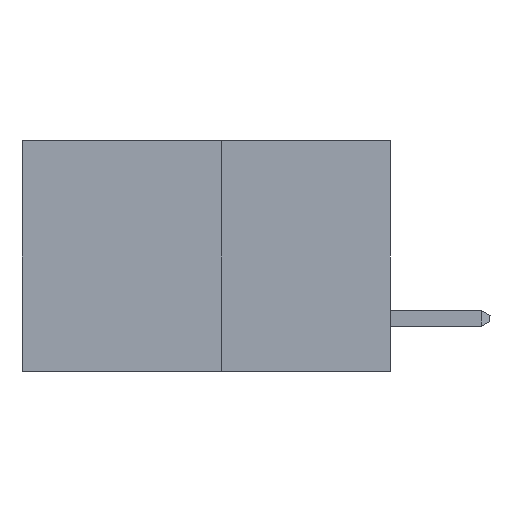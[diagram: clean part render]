
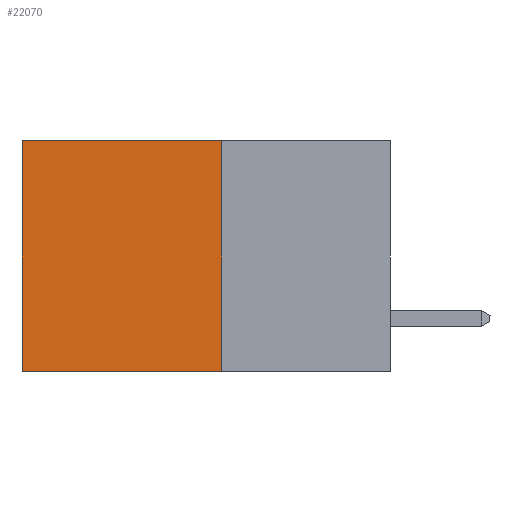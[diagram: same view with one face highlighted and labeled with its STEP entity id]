
A CAD part, left-side view. The second image highlights one B-rep face of the part: STEP entity #22070.
In plain terms, the highlighted planar face has unit normal (-1, 0, 0).
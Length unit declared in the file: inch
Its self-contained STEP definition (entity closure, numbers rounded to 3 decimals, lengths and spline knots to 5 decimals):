
#240 = CARTESIAN_POINT ( 'NONE',  ( 0.277, 0.27, -0.37 ) ) ;
#516 = ORIENTED_EDGE ( 'NONE', *, *, #8156, .T. ) ;
#986 = LINE ( 'NONE', #13013, #14407 ) ;
#2138 = ORIENTED_EDGE ( 'NONE', *, *, #2789, .F. ) ;
#2206 = DIRECTION ( 'NONE',  ( 1., 0., 0. ) ) ;
#2789 = EDGE_CURVE ( 'NONE', #14815, #9876, #11364, .T. ) ;
#3912 = EDGE_LOOP ( 'NONE', ( #7204, #5606, #2138, #516 ) ) ;
#3929 = CARTESIAN_POINT ( 'NONE',  ( 0.277, 0.59, 0. ) ) ;
#5356 = DIRECTION ( 'NONE',  ( 0., 1., 0. ) ) ;
#5384 = LINE ( 'NONE', #15681, #9479 ) ;
#5606 = ORIENTED_EDGE ( 'NONE', *, *, #20515, .F. ) ;
#6031 = VERTEX_POINT ( 'NONE', #10399 ) ;
#6675 = EDGE_CURVE ( 'NONE', #19231, #6031, #5384, .T. ) ;
#7046 = VECTOR ( 'NONE', #5356, 39.37008 ) ;
#7204 = ORIENTED_EDGE ( 'NONE', *, *, #6675, .T. ) ;
#8156 = EDGE_CURVE ( 'NONE', #14815, #19231, #986, .T. ) ;
#9479 = VECTOR ( 'NONE', #10471, 39.37008 ) ;
#9876 = VERTEX_POINT ( 'NONE', #240 ) ;
#10399 = CARTESIAN_POINT ( 'NONE',  ( 0.277, 0.59, -0.37 ) ) ;
#10471 = DIRECTION ( 'NONE',  ( 0., 0., -1. ) ) ;
#10573 = CARTESIAN_POINT ( 'NONE',  ( 0.277, 0.27, -0.37 ) ) ;
#10694 = DIRECTION ( 'NONE',  ( 0., 0., -1. ) ) ;
#11364 = LINE ( 'NONE', #10573, #19975 ) ;
#12669 = CARTESIAN_POINT ( 'NONE',  ( 0.277, 0.27, -0.37 ) ) ;
#13013 = CARTESIAN_POINT ( 'NONE',  ( 0.277, 0.27, 0. ) ) ;
#14146 = CARTESIAN_POINT ( 'NONE',  ( 0.277, 0.27, -0.37 ) ) ;
#14407 = VECTOR ( 'NONE', #14789, 39.37008 ) ;
#14439 = DIRECTION ( 'NONE',  ( 0., 0., -1. ) ) ;
#14789 = DIRECTION ( 'NONE',  ( 0., 1., 0. ) ) ;
#14815 = VERTEX_POINT ( 'NONE', #19083 ) ;
#15681 = CARTESIAN_POINT ( 'NONE',  ( 0.277, 0.59, -0.37 ) ) ;
#18353 = FACE_OUTER_BOUND ( 'NONE', #3912, .T. ) ;
#19083 = CARTESIAN_POINT ( 'NONE',  ( 0.277, 0.27, 0. ) ) ;
#19231 = VERTEX_POINT ( 'NONE', #3929 ) ;
#19975 = VECTOR ( 'NONE', #10694, 39.37008 ) ;
#20515 = EDGE_CURVE ( 'NONE', #9876, #6031, #21363, .T. ) ;
#21044 = AXIS2_PLACEMENT_3D ( 'NONE', #12669, #2206, #14439 ) ;
#21120 = PLANE ( 'NONE',  #21044 ) ;
#21363 = LINE ( 'NONE', #14146, #7046 ) ;
#22070 = ADVANCED_FACE ( 'NONE', ( #18353 ), #21120, .F. ) ;
